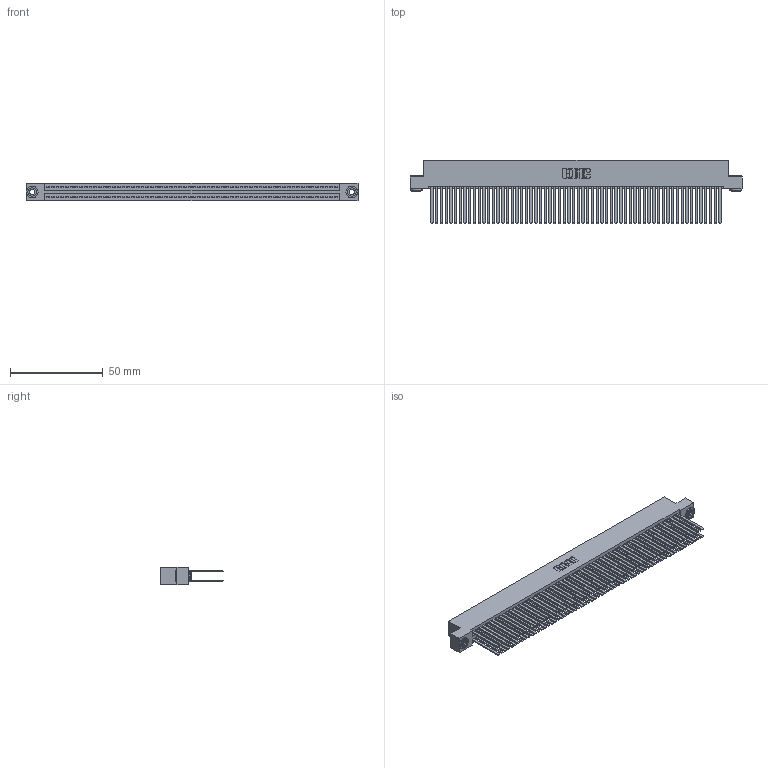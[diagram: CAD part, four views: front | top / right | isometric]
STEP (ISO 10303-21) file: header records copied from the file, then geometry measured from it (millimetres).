
FILE_DESCRIPTION (( 'STEP AP203' ), '1' );
FILE_NAME ('345-124-544-203.STEP', '2018-10-19T10:24:13', ( '' ), ( '' ), 'SwSTEP 2.0', 'SolidWorks 2016', '' );
FILE_SCHEMA (( 'CONFIG_CONTROL_DESIGN' ));
Length unit declared in the file: inch
Products named in the file (4): 345-124-544-203; 345-250-002_345-250-002-102; 345 Part_Flush Mounting Lugs - 0.156 Dia-TH; 345-292-001_345-293-144
Assembly tree (127 placements, depth 2):
  345-124-544-203
    345 Part_Flush Mounting Lugs - 0.156 Dia-TH
    345-292-001_345-293-144  x124
    345-250-002_345-250-002-102  x2
Bounding box: 178.69 x 33.96 x 9.4 mm (x, y, z)
Volume: 19301.3 mm3; surface area: 34217.5 mm2
Topology: 127 solids, 127 shells, 5620 faces, 16661 edges, 10938 vertices
Faces by surface type: plane 3686, cylinder 1926, cone 8
Entity records: 46420 total; most frequent: CARTESIAN_POINT 7735, ORIENTED_EDGE 7662, DIRECTION 6825, EDGE_CURVE 3831, LINE 3431, VECTOR 3431, VERTEX_POINT 2550, AXIS2_PLACEMENT_3D 1697
